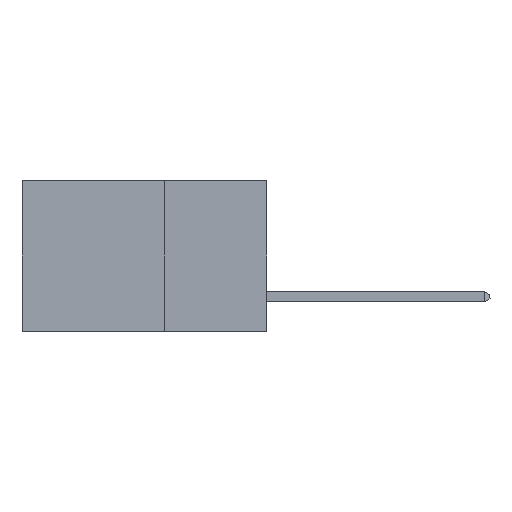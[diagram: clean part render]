
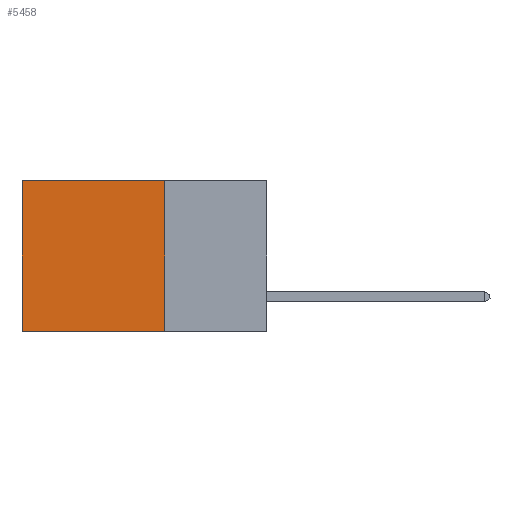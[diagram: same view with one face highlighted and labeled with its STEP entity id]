
A CAD part, left-side view. The second image highlights one B-rep face of the part: STEP entity #5458.
In plain terms, the highlighted planar face has unit normal (-1, 0, 0).
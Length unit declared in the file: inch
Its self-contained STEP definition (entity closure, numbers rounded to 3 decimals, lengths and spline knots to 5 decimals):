
#1107 = VECTOR ( 'NONE', #11114, 39.37008 ) ;
#1735 = CARTESIAN_POINT ( 'NONE',  ( 0.2875, 0.25, 0. ) ) ;
#1877 = ORIENTED_EDGE ( 'NONE', *, *, #11561, .T. ) ;
#2403 = LINE ( 'NONE', #10563, #8385 ) ;
#2661 = CARTESIAN_POINT ( 'NONE',  ( 0.2875, 0.25, 0. ) ) ;
#2753 = DIRECTION ( 'NONE',  ( 0., 0., -1. ) ) ;
#3645 = DIRECTION ( 'NONE',  ( 1., 0., 0. ) ) ;
#3790 = VECTOR ( 'NONE', #10314, 39.37008 ) ;
#3985 = ORIENTED_EDGE ( 'NONE', *, *, #5530, .T. ) ;
#4712 = VERTEX_POINT ( 'NONE', #12846 ) ;
#5458 = ADVANCED_FACE ( 'NONE', ( #13596 ), #12760, .F. ) ;
#5500 = CARTESIAN_POINT ( 'NONE',  ( 0.2875, 0.6, -0.37 ) ) ;
#5530 = EDGE_CURVE ( 'NONE', #13440, #4712, #6960, .T. ) ;
#6009 = CARTESIAN_POINT ( 'NONE',  ( 0.2875, 0.25, -0.37 ) ) ;
#6336 = EDGE_CURVE ( 'NONE', #13440, #11912, #9103, .T. ) ;
#6960 = LINE ( 'NONE', #7942, #3790 ) ;
#7382 = EDGE_CURVE ( 'NONE', #11912, #7660, #2403, .T. ) ;
#7660 = VERTEX_POINT ( 'NONE', #5500 ) ;
#7874 = LINE ( 'NONE', #8874, #1107 ) ;
#7887 = ORIENTED_EDGE ( 'NONE', *, *, #6336, .F. ) ;
#7942 = CARTESIAN_POINT ( 'NONE',  ( 0.2875, 0.25, 0. ) ) ;
#8385 = VECTOR ( 'NONE', #11652, 39.37008 ) ;
#8703 = CARTESIAN_POINT ( 'NONE',  ( 0.2875, 0.25, 0. ) ) ;
#8874 = CARTESIAN_POINT ( 'NONE',  ( 0.2875, 0.6, 0. ) ) ;
#9103 = LINE ( 'NONE', #2661, #13570 ) ;
#10314 = DIRECTION ( 'NONE',  ( 0., 1., 0. ) ) ;
#10563 = CARTESIAN_POINT ( 'NONE',  ( 0.2875, 0.25, -0.37 ) ) ;
#10595 = DIRECTION ( 'NONE',  ( 0., 0., -1. ) ) ;
#10931 = AXIS2_PLACEMENT_3D ( 'NONE', #8703, #3645, #10595 ) ;
#11114 = DIRECTION ( 'NONE',  ( 0., 0., -1. ) ) ;
#11561 = EDGE_CURVE ( 'NONE', #4712, #7660, #7874, .T. ) ;
#11652 = DIRECTION ( 'NONE',  ( 0., 1., 0. ) ) ;
#11912 = VERTEX_POINT ( 'NONE', #6009 ) ;
#12760 = PLANE ( 'NONE',  #10931 ) ;
#12846 = CARTESIAN_POINT ( 'NONE',  ( 0.2875, 0.6, 0. ) ) ;
#13232 = EDGE_LOOP ( 'NONE', ( #1877, #13779, #7887, #3985 ) ) ;
#13440 = VERTEX_POINT ( 'NONE', #1735 ) ;
#13570 = VECTOR ( 'NONE', #2753, 39.37008 ) ;
#13596 = FACE_OUTER_BOUND ( 'NONE', #13232, .T. ) ;
#13779 = ORIENTED_EDGE ( 'NONE', *, *, #7382, .F. ) ;
